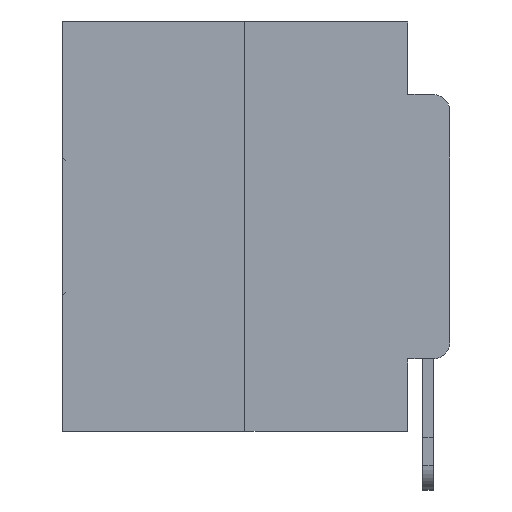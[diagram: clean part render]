
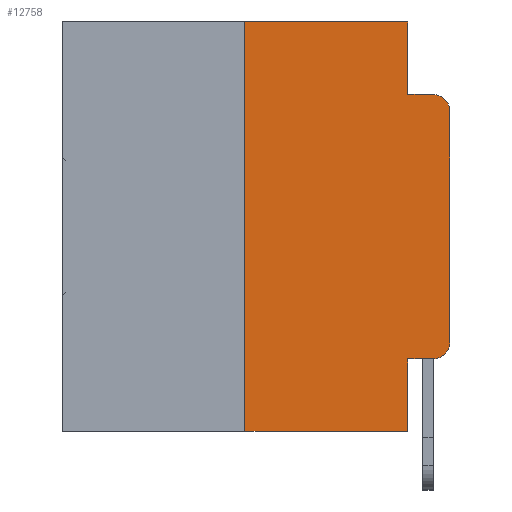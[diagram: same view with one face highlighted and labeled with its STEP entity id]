
A CAD part, left-side view. The second image highlights one B-rep face of the part: STEP entity #12758.
In plain terms, the highlighted planar face has unit normal (-1, 0, 0).
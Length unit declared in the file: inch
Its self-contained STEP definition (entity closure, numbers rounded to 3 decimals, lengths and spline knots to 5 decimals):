
#105 = DIRECTION ( 'NONE',  ( 0., 0., -1. ) ) ;
#493 = LINE ( 'NONE', #31314, #6612 ) ;
#1257 = CARTESIAN_POINT ( 'NONE',  ( 0., 0.051, -0.4115 ) ) ;
#1637 = VERTEX_POINT ( 'NONE', #14621 ) ;
#1725 = VECTOR ( 'NONE', #26715, 39.37008 ) ;
#1763 = VECTOR ( 'NONE', #6591, 39.37008 ) ;
#2616 = CARTESIAN_POINT ( 'NONE',  ( 0., 0.051, 0. ) ) ;
#2716 = CARTESIAN_POINT ( 'NONE',  ( 0., 0.02, -0.4115 ) ) ;
#2819 = VERTEX_POINT ( 'NONE', #20094 ) ;
#3000 = LINE ( 'NONE', #19365, #21741 ) ;
#3323 = VERTEX_POINT ( 'NONE', #29104 ) ;
#3860 = ORIENTED_EDGE ( 'NONE', *, *, #29093, .F. ) ;
#4081 = CARTESIAN_POINT ( 'NONE',  ( 0., 0.051, -0.5 ) ) ;
#4215 = VERTEX_POINT ( 'NONE', #2616 ) ;
#5562 = VERTEX_POINT ( 'NONE', #2716 ) ;
#6073 = EDGE_CURVE ( 'NONE', #1637, #9540, #28303, .T. ) ;
#6325 = VERTEX_POINT ( 'NONE', #1257 ) ;
#6591 = DIRECTION ( 'NONE',  ( 0., -1., 0. ) ) ;
#6612 = VECTOR ( 'NONE', #7738, 39.37008 ) ;
#6683 = EDGE_CURVE ( 'NONE', #6325, #15593, #8146, .T. ) ;
#7738 = DIRECTION ( 'NONE',  ( 0., -1., 0. ) ) ;
#7803 = LINE ( 'NONE', #31323, #1725 ) ;
#8146 = LINE ( 'NONE', #15123, #25638 ) ;
#8569 = PLANE ( 'NONE',  #28217 ) ;
#9426 = EDGE_CURVE ( 'NONE', #19829, #1637, #27565, .T. ) ;
#9447 = ORIENTED_EDGE ( 'NONE', *, *, #21842, .T. ) ;
#9458 = EDGE_CURVE ( 'NONE', #13503, #4215, #7803, .T. ) ;
#9540 = VERTEX_POINT ( 'NONE', #22297 ) ;
#10218 = ORIENTED_EDGE ( 'NONE', *, *, #20326, .T. ) ;
#10232 = CARTESIAN_POINT ( 'NONE',  ( 0., 0.02, -0.1085 ) ) ;
#10304 = EDGE_LOOP ( 'NONE', ( #21054, #15622, #3860, #17117, #24703, #30864, #12950, #14506, #9447, #10218 ) ) ;
#11013 = DIRECTION ( 'NONE',  ( 1., 0., 0. ) ) ;
#11265 = LINE ( 'NONE', #15758, #27926 ) ;
#12321 = CARTESIAN_POINT ( 'NONE',  ( 0., 0.25, 0. ) ) ;
#12758 = ADVANCED_FACE ( 'NONE', ( #23749 ), #8569, .F. ) ;
#12768 = DIRECTION ( 'NONE',  ( 0., 0., -1. ) ) ;
#12950 = ORIENTED_EDGE ( 'NONE', *, *, #19871, .T. ) ;
#13503 = VERTEX_POINT ( 'NONE', #19836 ) ;
#13600 = AXIS2_PLACEMENT_3D ( 'NONE', #28311, #14306, #30554 ) ;
#14306 = DIRECTION ( 'NONE',  ( -1., 0., 0. ) ) ;
#14406 = VECTOR ( 'NONE', #17414, 39.37008 ) ;
#14506 = ORIENTED_EDGE ( 'NONE', *, *, #6683, .F. ) ;
#14621 = CARTESIAN_POINT ( 'NONE',  ( 0., 0., -0.1085 ) ) ;
#14640 = DIRECTION ( 'NONE',  ( 0., -1., 0. ) ) ;
#15053 = EDGE_CURVE ( 'NONE', #2819, #13503, #23763, .T. ) ;
#15123 = CARTESIAN_POINT ( 'NONE',  ( 0., 0.051, 0. ) ) ;
#15593 = VERTEX_POINT ( 'NONE', #4081 ) ;
#15622 = ORIENTED_EDGE ( 'NONE', *, *, #6073, .T. ) ;
#15758 = CARTESIAN_POINT ( 'NONE',  ( 0., 0.051, 0. ) ) ;
#17117 = ORIENTED_EDGE ( 'NONE', *, *, #22816, .F. ) ;
#17414 = DIRECTION ( 'NONE',  ( 0., 0., 1. ) ) ;
#18107 = DIRECTION ( 'NONE',  ( 0., 0., -1. ) ) ;
#18348 = VECTOR ( 'NONE', #28781, 39.37008 ) ;
#18786 = CARTESIAN_POINT ( 'NONE',  ( 0., 0.473, -0.5 ) ) ;
#19365 = CARTESIAN_POINT ( 'NONE',  ( 0., 0.051, -0.4115 ) ) ;
#19711 = CARTESIAN_POINT ( 'NONE',  ( 0., 0., 0. ) ) ;
#19829 = VERTEX_POINT ( 'NONE', #23190 ) ;
#19836 = CARTESIAN_POINT ( 'NONE',  ( 0., 0.25, 0. ) ) ;
#19871 = EDGE_CURVE ( 'NONE', #2819, #15593, #27598, .T. ) ;
#20094 = CARTESIAN_POINT ( 'NONE',  ( 0., 0.25, -0.5 ) ) ;
#20326 = EDGE_CURVE ( 'NONE', #5562, #19829, #26218, .T. ) ;
#21054 = ORIENTED_EDGE ( 'NONE', *, *, #9426, .T. ) ;
#21741 = VECTOR ( 'NONE', #14640, 39.37008 ) ;
#21842 = EDGE_CURVE ( 'NONE', #6325, #5562, #3000, .T. ) ;
#22297 = CARTESIAN_POINT ( 'NONE',  ( 0., 0.02, -0.0885 ) ) ;
#22816 = EDGE_CURVE ( 'NONE', #4215, #3323, #11265, .T. ) ;
#23190 = CARTESIAN_POINT ( 'NONE',  ( 0., 0., -0.3915 ) ) ;
#23749 = FACE_OUTER_BOUND ( 'NONE', #10304, .T. ) ;
#23763 = LINE ( 'NONE', #12321, #18348 ) ;
#24287 = AXIS2_PLACEMENT_3D ( 'NONE', #10232, #26851, #12768 ) ;
#24703 = ORIENTED_EDGE ( 'NONE', *, *, #9458, .F. ) ;
#25216 = CARTESIAN_POINT ( 'NONE',  ( 0., 0.473, 0. ) ) ;
#25638 = VECTOR ( 'NONE', #105, 39.37008 ) ;
#26218 = CIRCLE ( 'NONE', #13600, 0.02 ) ;
#26715 = DIRECTION ( 'NONE',  ( 0., -1., 0. ) ) ;
#26851 = DIRECTION ( 'NONE',  ( -1., 0., 0. ) ) ;
#27565 = LINE ( 'NONE', #19711, #14406 ) ;
#27590 = DIRECTION ( 'NONE',  ( 0., 0., -1. ) ) ;
#27598 = LINE ( 'NONE', #18786, #1763 ) ;
#27926 = VECTOR ( 'NONE', #18107, 39.37008 ) ;
#28217 = AXIS2_PLACEMENT_3D ( 'NONE', #25216, #11013, #27590 ) ;
#28303 = CIRCLE ( 'NONE', #24287, 0.02 ) ;
#28311 = CARTESIAN_POINT ( 'NONE',  ( 0., 0.02, -0.3915 ) ) ;
#28781 = DIRECTION ( 'NONE',  ( 0., 0., 1. ) ) ;
#29093 = EDGE_CURVE ( 'NONE', #3323, #9540, #493, .T. ) ;
#29104 = CARTESIAN_POINT ( 'NONE',  ( 0., 0.051, -0.0885 ) ) ;
#30554 = DIRECTION ( 'NONE',  ( 0., 0., -1. ) ) ;
#30864 = ORIENTED_EDGE ( 'NONE', *, *, #15053, .F. ) ;
#31314 = CARTESIAN_POINT ( 'NONE',  ( 0., 0.051, -0.0885 ) ) ;
#31323 = CARTESIAN_POINT ( 'NONE',  ( 0., 0.473, 0. ) ) ;
